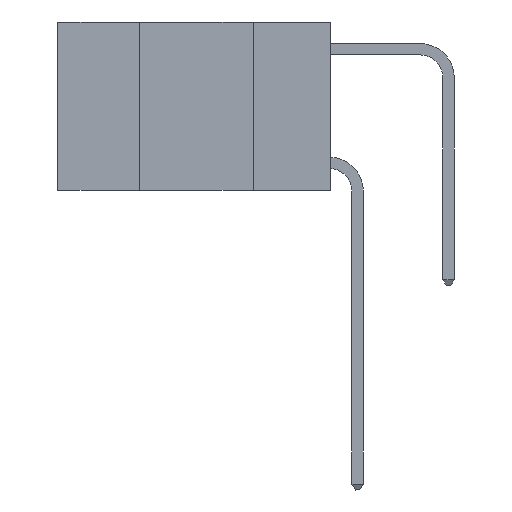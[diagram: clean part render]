
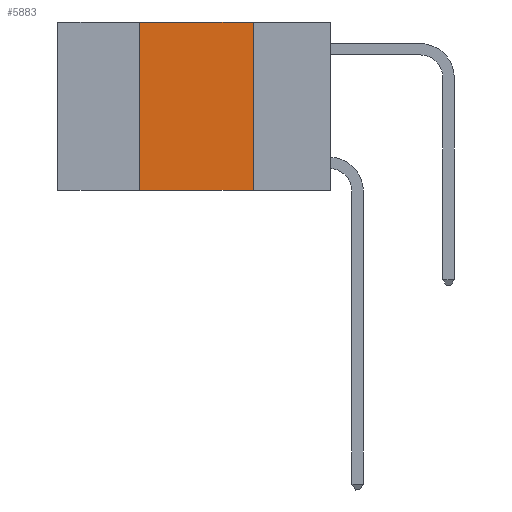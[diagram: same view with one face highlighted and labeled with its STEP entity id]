
A CAD part, left-side view. The second image highlights one B-rep face of the part: STEP entity #5883.
In plain terms, the highlighted planar face has unit normal (-1, 0, 0).
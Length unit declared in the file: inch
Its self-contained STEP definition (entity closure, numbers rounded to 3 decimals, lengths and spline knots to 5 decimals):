
#1204 = VECTOR ( 'NONE', #2620, 39.37008 ) ;
#1494 = VERTEX_POINT ( 'NONE', #8083 ) ;
#1815 = DIRECTION ( 'NONE',  ( 0., 0., -1. ) ) ;
#1876 = LINE ( 'NONE', #3119, #14852 ) ;
#2620 = DIRECTION ( 'NONE',  ( 0., -1., 0. ) ) ;
#2630 = VERTEX_POINT ( 'NONE', #10278 ) ;
#3119 = CARTESIAN_POINT ( 'NONE',  ( 0., 0.6, -0.37 ) ) ;
#3147 = CARTESIAN_POINT ( 'NONE',  ( 0., 0.6, 0. ) ) ;
#3460 = AXIS2_PLACEMENT_3D ( 'NONE', #5701, #11132, #17421 ) ;
#3663 = CARTESIAN_POINT ( 'NONE',  ( 0., 0.42, 0. ) ) ;
#3939 = LINE ( 'NONE', #3147, #1204 ) ;
#4645 = DIRECTION ( 'NONE',  ( 0., -1., 0. ) ) ;
#5701 = CARTESIAN_POINT ( 'NONE',  ( 0., 0.6, 0. ) ) ;
#5847 = EDGE_CURVE ( 'NONE', #16302, #1494, #13363, .T. ) ;
#5883 = ADVANCED_FACE ( 'NONE', ( #7105 ), #18810, .F. ) ;
#6291 = DIRECTION ( 'NONE',  ( 0., 0., 1. ) ) ;
#6327 = EDGE_CURVE ( 'NONE', #2630, #16302, #3939, .T. ) ;
#7105 = FACE_OUTER_BOUND ( 'NONE', #14496, .T. ) ;
#7751 = LINE ( 'NONE', #3663, #7996 ) ;
#7996 = VECTOR ( 'NONE', #6291, 39.37008 ) ;
#8083 = CARTESIAN_POINT ( 'NONE',  ( 0., 0.17, -0.37 ) ) ;
#9336 = CARTESIAN_POINT ( 'NONE',  ( 0., 0.17, 0. ) ) ;
#10278 = CARTESIAN_POINT ( 'NONE',  ( 0., 0.42, 0. ) ) ;
#10485 = CARTESIAN_POINT ( 'NONE',  ( 0., 0.17, 0. ) ) ;
#10608 = VERTEX_POINT ( 'NONE', #12745 ) ;
#11132 = DIRECTION ( 'NONE',  ( 1., 0., 0. ) ) ;
#12745 = CARTESIAN_POINT ( 'NONE',  ( 0., 0.42, -0.37 ) ) ;
#12900 = VECTOR ( 'NONE', #1815, 39.37008 ) ;
#13363 = LINE ( 'NONE', #10485, #12900 ) ;
#13876 = ORIENTED_EDGE ( 'NONE', *, *, #18435, .F. ) ;
#14418 = ORIENTED_EDGE ( 'NONE', *, *, #6327, .F. ) ;
#14464 = EDGE_CURVE ( 'NONE', #10608, #1494, #1876, .T. ) ;
#14496 = EDGE_LOOP ( 'NONE', ( #16669, #14418, #13876, #15428 ) ) ;
#14852 = VECTOR ( 'NONE', #4645, 39.37008 ) ;
#15428 = ORIENTED_EDGE ( 'NONE', *, *, #14464, .T. ) ;
#16302 = VERTEX_POINT ( 'NONE', #9336 ) ;
#16669 = ORIENTED_EDGE ( 'NONE', *, *, #5847, .F. ) ;
#17421 = DIRECTION ( 'NONE',  ( 0., 0., -1. ) ) ;
#18435 = EDGE_CURVE ( 'NONE', #10608, #2630, #7751, .T. ) ;
#18810 = PLANE ( 'NONE',  #3460 ) ;
